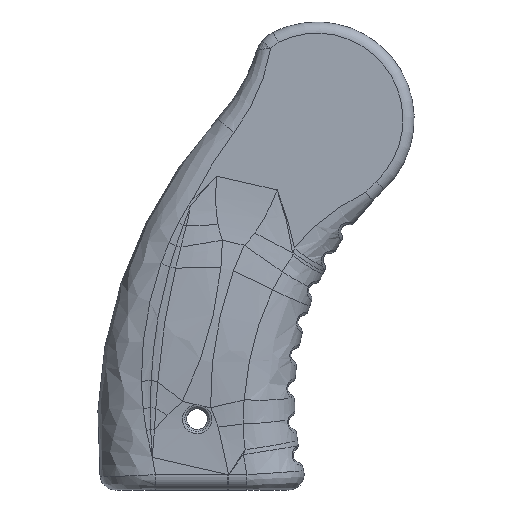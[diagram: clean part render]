
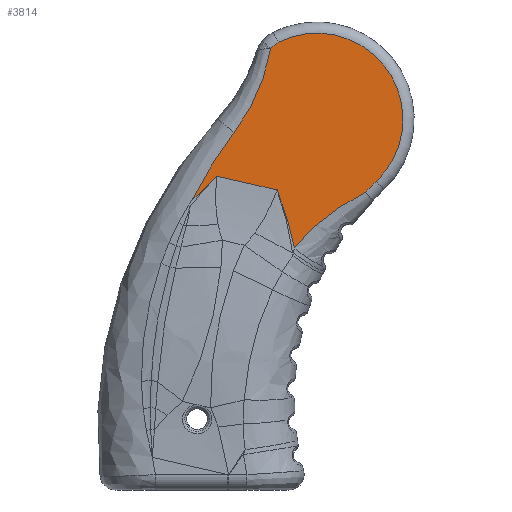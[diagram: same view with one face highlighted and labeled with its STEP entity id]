
A CAD part, front view. The second image highlights one B-rep face of the part: STEP entity #3814.
In plain terms, the highlighted planar face has unit normal (0, -1, 0).
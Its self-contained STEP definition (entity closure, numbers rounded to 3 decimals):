
#37=PLANE('',#4168);
#89=LINE('',#8476,#187);
#187=VECTOR('',#4752,10.);
#569=FACE_OUTER_BOUND('',#832,.T.);
#832=EDGE_LOOP('',(#2993,#2994,#2995,#2996,#2997,#2998,#2999,#3000,#3001,
#3002));
#1057=B_SPLINE_CURVE_WITH_KNOTS('',3,(#7180,#7181,#7182,#7183,#7184),
 .UNSPECIFIED.,.F.,.F.,(4,1,4),(0.198,0.358,0.476),
 .UNSPECIFIED.);
#1104=B_SPLINE_CURVE_WITH_KNOTS('',3,(#8118,#8119,#8120,#8121,#8122,#8123),
 .UNSPECIFIED.,.F.,.F.,(4,2,4),(0.142,0.227,0.228),
 .UNSPECIFIED.);
#1115=B_SPLINE_CURVE_WITH_KNOTS('',3,(#8365,#8366,#8367,#8368,#8369,#8370),
 .UNSPECIFIED.,.F.,.F.,(4,2,4),(-0.507,0.,0.005),
 .UNSPECIFIED.);
#1119=B_SPLINE_CURVE_WITH_KNOTS('',3,(#8477,#8478,#8479,#8480,#8481,#8482),
 .UNSPECIFIED.,.F.,.F.,(4,2,4),(-1.76,-1.755,-0.68),
 .UNSPECIFIED.);
#1120=B_SPLINE_CURVE_WITH_KNOTS('',3,(#8490,#8491,#8492,#8493,#8494,#8495),
 .UNSPECIFIED.,.F.,.F.,(4,2,4),(-0.338,0.,1.319),
 .UNSPECIFIED.);
#1121=B_SPLINE_CURVE_WITH_KNOTS('',3,(#8496,#8497,#8498,#8499),
 .UNSPECIFIED.,.F.,.F.,(4,4),(1.319,2.734),
 .UNSPECIFIED.);
#1410=CIRCLE('',#4169,53.538);
#1411=CIRCLE('',#4170,15.352);
#1412=CIRCLE('',#4171,4.);
#1648=VERTEX_POINT('',#7099);
#1649=VERTEX_POINT('',#7179);
#1696=VERTEX_POINT('',#8103);
#1697=VERTEX_POINT('',#8117);
#1704=VERTEX_POINT('',#8328);
#1707=VERTEX_POINT('',#8475);
#1708=VERTEX_POINT('',#8483);
#1709=VERTEX_POINT('',#8485);
#1710=VERTEX_POINT('',#8487);
#1711=VERTEX_POINT('',#8489);
#2076=EDGE_CURVE('',#1649,#1648,#1057,.T.);
#2150=EDGE_CURVE('',#1696,#1697,#1104,.T.);
#2168=EDGE_CURVE('',#1696,#1704,#1115,.T.);
#2176=EDGE_CURVE('',#1704,#1707,#89,.T.);
#2177=EDGE_CURVE('',#1707,#1649,#1119,.T.);
#2178=EDGE_CURVE('',#1648,#1708,#1410,.T.);
#2179=EDGE_CURVE('',#1708,#1709,#1411,.T.);
#2180=EDGE_CURVE('',#1709,#1710,#1412,.T.);
#2181=EDGE_CURVE('',#1710,#1711,#1120,.T.);
#2182=EDGE_CURVE('',#1711,#1697,#1121,.T.);
#2993=ORIENTED_EDGE('',*,*,#2150,.F.);
#2994=ORIENTED_EDGE('',*,*,#2168,.T.);
#2995=ORIENTED_EDGE('',*,*,#2176,.T.);
#2996=ORIENTED_EDGE('',*,*,#2177,.T.);
#2997=ORIENTED_EDGE('',*,*,#2076,.T.);
#2998=ORIENTED_EDGE('',*,*,#2178,.T.);
#2999=ORIENTED_EDGE('',*,*,#2179,.T.);
#3000=ORIENTED_EDGE('',*,*,#2180,.T.);
#3001=ORIENTED_EDGE('',*,*,#2181,.T.);
#3002=ORIENTED_EDGE('',*,*,#2182,.T.);
#3814=ADVANCED_FACE('',(#569),#37,.F.);
#4168=AXIS2_PLACEMENT_3D('',#8474,#4750,#4751);
#4169=AXIS2_PLACEMENT_3D('',#8484,#4753,#4754);
#4170=AXIS2_PLACEMENT_3D('',#8486,#4755,#4756);
#4171=AXIS2_PLACEMENT_3D('',#8488,#4757,#4758);
#4750=DIRECTION('center_axis',(0.,1.,0.));
#4751=DIRECTION('ref_axis',(1.,0.,0.));
#4752=DIRECTION('',(0.975,0.,-0.222));
#4753=DIRECTION('center_axis',(0.,1.,0.));
#4754=DIRECTION('ref_axis',(0.69,0.,-0.724));
#4755=DIRECTION('center_axis',(0.,-1.,0.));
#4756=DIRECTION('ref_axis',(0.78,0.,0.626));
#4757=DIRECTION('center_axis',(0.,-1.,0.));
#4758=DIRECTION('ref_axis',(-0.63,0.,0.777));
#7099=CARTESIAN_POINT('',(30.358,-6.75,50.211));
#7179=CARTESIAN_POINT('',(17.65,-6.75,40.273));
#7180=CARTESIAN_POINT('Ctrl Pts',(17.65,-6.75,40.273));
#7181=CARTESIAN_POINT('Ctrl Pts',(19.673,-6.75,42.723));
#7182=CARTESIAN_POINT('Ctrl Pts',(23.702,-6.75,46.489));
#7183=CARTESIAN_POINT('Ctrl Pts',(28.354,-6.75,49.219));
#7184=CARTESIAN_POINT('Ctrl Pts',(30.358,-6.75,50.211));
#8103=CARTESIAN_POINT('',(0.145,-6.75,49.461));
#8117=CARTESIAN_POINT('',(-0.54,-6.75,48.943));
#8118=CARTESIAN_POINT('Ctrl Pts',(0.145,-6.75,49.461));
#8119=CARTESIAN_POINT('Ctrl Pts',(-0.074,-6.75,49.279));
#8120=CARTESIAN_POINT('Ctrl Pts',(-0.302,-6.75,49.105));
#8121=CARTESIAN_POINT('Ctrl Pts',(-0.536,-6.75,48.946));
#8122=CARTESIAN_POINT('Ctrl Pts',(-0.538,-6.75,48.945));
#8123=CARTESIAN_POINT('Ctrl Pts',(-0.54,-6.75,48.943));
#8328=CARTESIAN_POINT('',(3.772,-6.75,53.09));
#8365=CARTESIAN_POINT('Ctrl Pts',(0.145,-6.75,49.461));
#8366=CARTESIAN_POINT('Ctrl Pts',(1.291,-6.75,50.711));
#8367=CARTESIAN_POINT('Ctrl Pts',(2.493,-6.75,51.911));
#8368=CARTESIAN_POINT('Ctrl Pts',(3.749,-6.75,53.068));
#8369=CARTESIAN_POINT('Ctrl Pts',(3.76,-6.75,53.079));
#8370=CARTESIAN_POINT('Ctrl Pts',(3.772,-6.75,53.09));
#8474=CARTESIAN_POINT('Origin',(51.519,-6.75,24.406));
#8475=CARTESIAN_POINT('',(14.585,-6.75,50.63));
#8476=CARTESIAN_POINT('',(55.495,-6.75,41.32));
#8477=CARTESIAN_POINT('Ctrl Pts',(14.585,-6.75,50.63));
#8478=CARTESIAN_POINT('Ctrl Pts',(14.591,-6.75,50.615));
#8479=CARTESIAN_POINT('Ctrl Pts',(14.597,-6.75,50.599));
#8480=CARTESIAN_POINT('Ctrl Pts',(15.928,-6.75,47.255));
#8481=CARTESIAN_POINT('Ctrl Pts',(16.977,-6.75,43.794));
#8482=CARTESIAN_POINT('Ctrl Pts',(17.65,-6.75,40.273));
#8483=CARTESIAN_POINT('',(32.265,-6.75,52.123));
#8484=CARTESIAN_POINT('Origin',(69.213,-6.75,13.378));
#8485=CARTESIAN_POINT('',(14.769,-6.75,76.947));
#8486=CARTESIAN_POINT('Origin',(21.67,-6.75,63.234));
#8487=CARTESIAN_POINT('',(13.442,-6.75,75.871));
#8488=CARTESIAN_POINT('Origin',(16.567,-6.75,73.374));
#8489=CARTESIAN_POINT('',(6.906,-6.75,60.88));
#8490=CARTESIAN_POINT('Ctrl Pts',(13.442,-6.75,75.871));
#8491=CARTESIAN_POINT('Ctrl Pts',(13.25,-6.75,74.759));
#8492=CARTESIAN_POINT('Ctrl Pts',(13.003,-6.75,73.662));
#8493=CARTESIAN_POINT('Ctrl Pts',(11.537,-6.75,68.359));
#8494=CARTESIAN_POINT('Ctrl Pts',(9.549,-6.75,64.371));
#8495=CARTESIAN_POINT('Ctrl Pts',(6.906,-6.75,60.88));
#8496=CARTESIAN_POINT('Ctrl Pts',(6.906,-6.75,60.88));
#8497=CARTESIAN_POINT('Ctrl Pts',(4.072,-6.75,57.136));
#8498=CARTESIAN_POINT('Ctrl Pts',(1.577,-6.75,53.135));
#8499=CARTESIAN_POINT('Ctrl Pts',(-0.537,-6.75,48.942));
